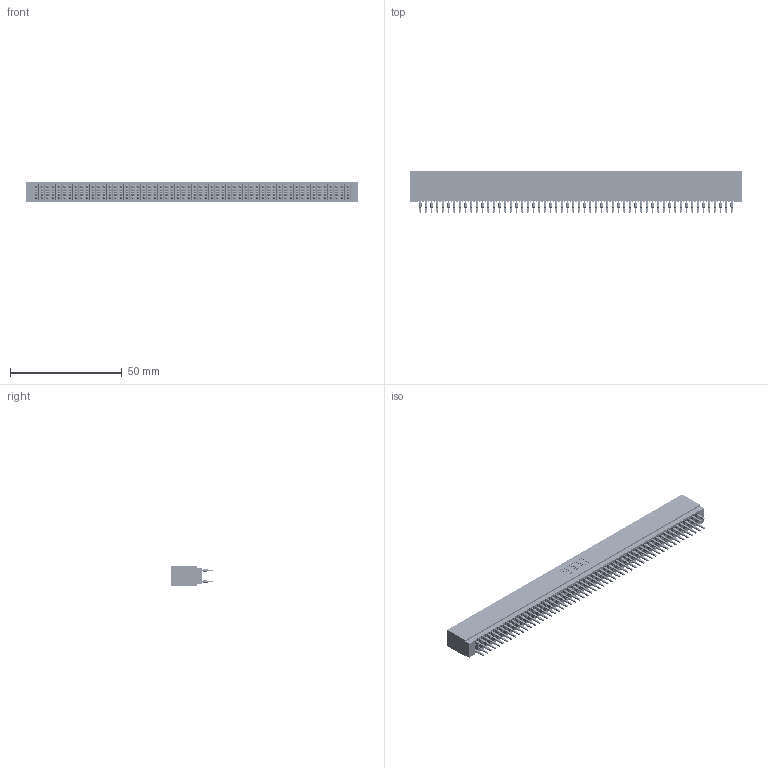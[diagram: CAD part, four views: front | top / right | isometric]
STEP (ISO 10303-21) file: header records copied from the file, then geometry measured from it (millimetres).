
FILE_DESCRIPTION (( 'STEP AP203' ), '1' );
FILE_NAME ('725-112-560-201.STEP', '2026-02-24T20:38:40', ( '' ), ( '' ), 'SwSTEP 2.0', 'SolidWorks 2023', '' );
FILE_SCHEMA (( 'CONFIG_CONTROL_DESIGN' ));
Products named in the file (3): 745-292-001_560; 725 Part_Insulator Option - 01; 725-112-560-201
Assembly tree (113 placements, depth 2):
  725-112-560-201
    725 Part_Insulator Option - 01
    745-292-001_560  x112
Bounding box: 148.84 x 18.8 x 8.89 mm (x, y, z)
Volume: 12146.7 mm3; surface area: 27720.7 mm2
Topology: 113 solids, 113 shells, 11127 faces, 30438 edges, 19320 vertices
Faces by surface type: plane 5767, cylinder 2448, bspline 2240, torus 672
Entity records: 92653 total; most frequent: CARTESIAN_POINT 16569, ORIENTED_EDGE 16032, DIRECTION 14000, EDGE_CURVE 8016, VECTOR 7490, LINE 7490, VERTEX_POINT 5112, AXIS2_PLACEMENT_3D 3255
